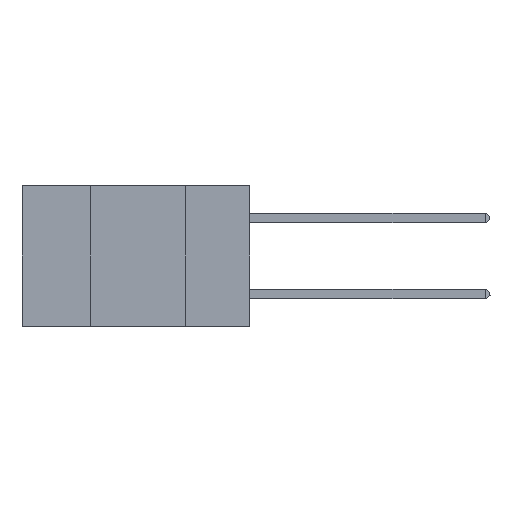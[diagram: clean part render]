
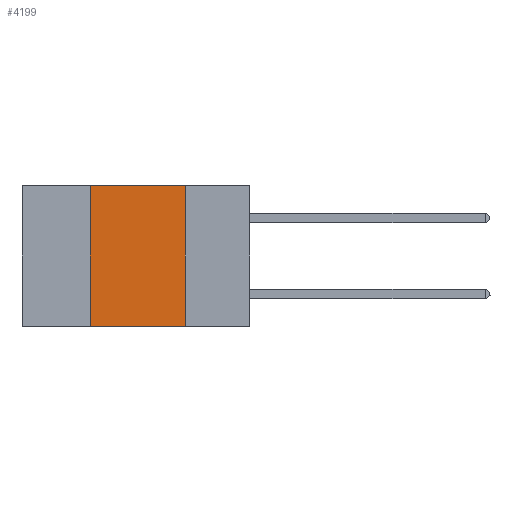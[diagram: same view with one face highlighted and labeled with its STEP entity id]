
A CAD part, left-side view. The second image highlights one B-rep face of the part: STEP entity #4199.
In plain terms, the highlighted planar face has unit normal (-1, 0, 0).
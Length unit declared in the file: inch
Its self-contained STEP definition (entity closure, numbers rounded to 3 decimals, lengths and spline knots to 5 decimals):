
#493 = EDGE_CURVE ( 'NONE', #5532, #3885, #13566, .T. ) ;
#1541 = VECTOR ( 'NONE', #20683, 39.37008 ) ;
#2544 = CARTESIAN_POINT ( 'NONE',  ( 0., 0.17, -0.37 ) ) ;
#3885 = VERTEX_POINT ( 'NONE', #2544 ) ;
#4199 = ADVANCED_FACE ( 'NONE', ( #12598 ), #14946, .F. ) ;
#4337 = ORIENTED_EDGE ( 'NONE', *, *, #19110, .F. ) ;
#4542 = CARTESIAN_POINT ( 'NONE',  ( 0., 0.17, 0. ) ) ;
#5532 = VERTEX_POINT ( 'NONE', #6420 ) ;
#5539 = LINE ( 'NONE', #25569, #15111 ) ;
#6420 = CARTESIAN_POINT ( 'NONE',  ( 0., 0.42, -0.37 ) ) ;
#7881 = ORIENTED_EDGE ( 'NONE', *, *, #27976, .F. ) ;
#9076 = AXIS2_PLACEMENT_3D ( 'NONE', #10986, #17528, #26804 ) ;
#9637 = LINE ( 'NONE', #13437, #27343 ) ;
#10377 = ORIENTED_EDGE ( 'NONE', *, *, #25210, .F. ) ;
#10986 = CARTESIAN_POINT ( 'NONE',  ( 0., 0.6, 0. ) ) ;
#11352 = CARTESIAN_POINT ( 'NONE',  ( 0., 0.42, 0. ) ) ;
#11665 = DIRECTION ( 'NONE',  ( 0., -1., 0. ) ) ;
#12291 = DIRECTION ( 'NONE',  ( 0., 0., -1. ) ) ;
#12598 = FACE_OUTER_BOUND ( 'NONE', #18758, .T. ) ;
#12604 = LINE ( 'NONE', #11352, #25731 ) ;
#13437 = CARTESIAN_POINT ( 'NONE',  ( 0., 0.6, 0. ) ) ;
#13566 = LINE ( 'NONE', #25099, #1541 ) ;
#14946 = PLANE ( 'NONE',  #9076 ) ;
#15111 = VECTOR ( 'NONE', #12291, 39.37008 ) ;
#17528 = DIRECTION ( 'NONE',  ( 1., 0., 0. ) ) ;
#18758 = EDGE_LOOP ( 'NONE', ( #10377, #7881, #4337, #21334 ) ) ;
#19110 = EDGE_CURVE ( 'NONE', #5532, #20290, #12604, .T. ) ;
#20290 = VERTEX_POINT ( 'NONE', #25435 ) ;
#20683 = DIRECTION ( 'NONE',  ( 0., -1., 0. ) ) ;
#21334 = ORIENTED_EDGE ( 'NONE', *, *, #493, .T. ) ;
#25099 = CARTESIAN_POINT ( 'NONE',  ( 0., 0.6, -0.37 ) ) ;
#25210 = EDGE_CURVE ( 'NONE', #26135, #3885, #5539, .T. ) ;
#25435 = CARTESIAN_POINT ( 'NONE',  ( 0., 0.42, 0. ) ) ;
#25569 = CARTESIAN_POINT ( 'NONE',  ( 0., 0.17, 0. ) ) ;
#25731 = VECTOR ( 'NONE', #27467, 39.37008 ) ;
#26135 = VERTEX_POINT ( 'NONE', #4542 ) ;
#26804 = DIRECTION ( 'NONE',  ( 0., 0., -1. ) ) ;
#27343 = VECTOR ( 'NONE', #11665, 39.37008 ) ;
#27467 = DIRECTION ( 'NONE',  ( 0., 0., 1. ) ) ;
#27976 = EDGE_CURVE ( 'NONE', #20290, #26135, #9637, .T. ) ;
